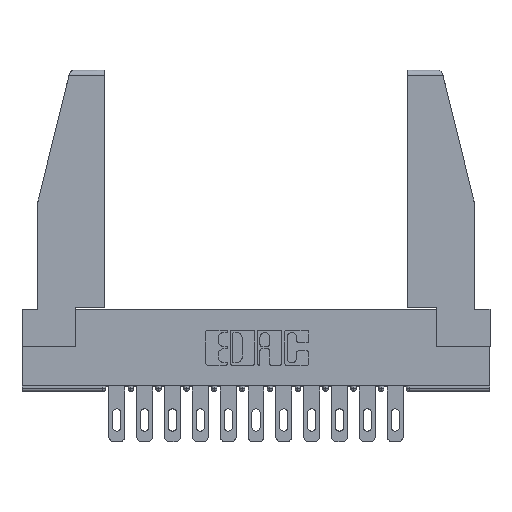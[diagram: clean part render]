
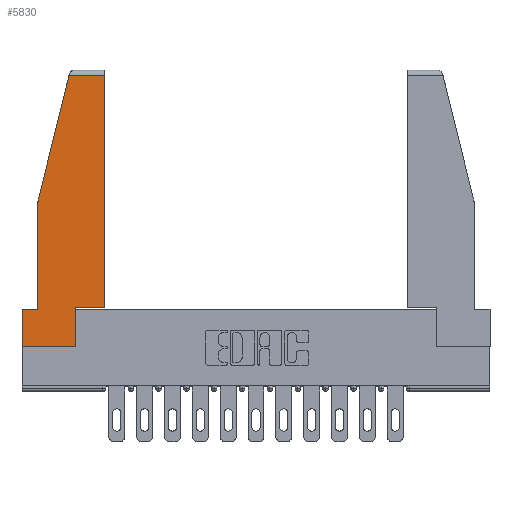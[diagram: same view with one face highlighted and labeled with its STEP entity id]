
A CAD part, top view. The second image highlights one B-rep face of the part: STEP entity #5830.
In plain terms, the highlighted planar face has unit normal (0, 0, 1).
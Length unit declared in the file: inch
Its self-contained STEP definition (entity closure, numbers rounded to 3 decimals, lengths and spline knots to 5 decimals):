
#15 = EDGE_CURVE ( 'NONE', #6433, #5348, #11458, .T. ) ;
#330 = DIRECTION ( 'NONE',  ( -1., 0., 0. ) ) ;
#631 = CARTESIAN_POINT ( 'NONE',  ( 0.297, 0., 0. ) ) ;
#1104 = DIRECTION ( 'NONE',  ( 1., 0., 0. ) ) ;
#1249 = ORIENTED_EDGE ( 'NONE', *, *, #12569, .T. ) ;
#1342 = CARTESIAN_POINT ( 'NONE',  ( 0., 0.21, 0. ) ) ;
#1896 = ORIENTED_EDGE ( 'NONE', *, *, #3203, .T. ) ;
#2034 = VECTOR ( 'NONE', #15187, 39.37008 ) ;
#2132 = VERTEX_POINT ( 'NONE', #4320 ) ;
#2552 = LINE ( 'NONE', #7394, #5013 ) ;
#2830 = VECTOR ( 'NONE', #11632, 39.37008 ) ;
#2908 = LINE ( 'NONE', #9413, #16476 ) ;
#3203 = EDGE_CURVE ( 'NONE', #11851, #7117, #3921, .T. ) ;
#3472 = VECTOR ( 'NONE', #7730, 39.37008 ) ;
#3849 = AXIS2_PLACEMENT_3D ( 'NONE', #8114, #9513, #1104 ) ;
#3921 = LINE ( 'NONE', #13723, #15728 ) ;
#4055 = EDGE_LOOP ( 'NONE', ( #10282, #1896, #13260, #15334, #10224, #13659, #14920, #1249, #7175 ) ) ;
#4320 = CARTESIAN_POINT ( 'NONE',  ( 0.297, 0., 0. ) ) ;
#4621 = VECTOR ( 'NONE', #14082, 39.37008 ) ;
#4877 = CARTESIAN_POINT ( 'NONE',  ( 0.461, 0.223, 0. ) ) ;
#5013 = VECTOR ( 'NONE', #330, 39.37008 ) ;
#5178 = CARTESIAN_POINT ( 'NONE',  ( 0.297, 0.223, 0. ) ) ;
#5245 = VERTEX_POINT ( 'NONE', #5178 ) ;
#5348 = VERTEX_POINT ( 'NONE', #12606 ) ;
#5524 = VECTOR ( 'NONE', #9646, 39.37008 ) ;
#5820 = CARTESIAN_POINT ( 'NONE',  ( 0.2636, 1.52, 0. ) ) ;
#5830 = ADVANCED_FACE ( 'NONE', ( #17944 ), #6725, .T. ) ;
#6433 = VERTEX_POINT ( 'NONE', #1342 ) ;
#6725 = PLANE ( 'NONE',  #3849 ) ;
#7117 = VERTEX_POINT ( 'NONE', #5820 ) ;
#7175 = ORIENTED_EDGE ( 'NONE', *, *, #15026, .T. ) ;
#7382 = CARTESIAN_POINT ( 'NONE',  ( 0.086, 0.8, 0. ) ) ;
#7394 = CARTESIAN_POINT ( 'NONE',  ( 0., 0.21, 0. ) ) ;
#7730 = DIRECTION ( 'NONE',  ( 0., -1., 0. ) ) ;
#8114 = CARTESIAN_POINT ( 'NONE',  ( 0., 0., 0. ) ) ;
#8249 = CARTESIAN_POINT ( 'NONE',  ( 0.297, 0.223, 0. ) ) ;
#8479 = EDGE_CURVE ( 'NONE', #7117, #10100, #2908, .T. ) ;
#8643 = VERTEX_POINT ( 'NONE', #9326 ) ;
#8775 = CARTESIAN_POINT ( 'NONE',  ( 0.461, 0.223, 0. ) ) ;
#9326 = CARTESIAN_POINT ( 'NONE',  ( 0.086, 0.21, 0. ) ) ;
#9413 = CARTESIAN_POINT ( 'NONE',  ( 0.271, 1.55, 0. ) ) ;
#9513 = DIRECTION ( 'NONE',  ( 0., 0., 1. ) ) ;
#9646 = DIRECTION ( 'NONE',  ( 1., 0., 0. ) ) ;
#10100 = VERTEX_POINT ( 'NONE', #7382 ) ;
#10139 = EDGE_CURVE ( 'NONE', #17479, #11851, #10907, .T. ) ;
#10224 = ORIENTED_EDGE ( 'NONE', *, *, #11218, .T. ) ;
#10282 = ORIENTED_EDGE ( 'NONE', *, *, #10139, .T. ) ;
#10804 = LINE ( 'NONE', #631, #12809 ) ;
#10900 = EDGE_CURVE ( 'NONE', #10100, #8643, #13528, .T. ) ;
#10907 = LINE ( 'NONE', #8775, #2830 ) ;
#11218 = EDGE_CURVE ( 'NONE', #8643, #6433, #2552, .T. ) ;
#11458 = LINE ( 'NONE', #13712, #2034 ) ;
#11632 = DIRECTION ( 'NONE',  ( 0., 1., 0. ) ) ;
#11851 = VERTEX_POINT ( 'NONE', #15563 ) ;
#12170 = DIRECTION ( 'NONE',  ( -0.239, -0.971, 0. ) ) ;
#12569 = EDGE_CURVE ( 'NONE', #2132, #5245, #10804, .T. ) ;
#12606 = CARTESIAN_POINT ( 'NONE',  ( 0., 0., 0. ) ) ;
#12809 = VECTOR ( 'NONE', #17321, 39.37008 ) ;
#13260 = ORIENTED_EDGE ( 'NONE', *, *, #8479, .T. ) ;
#13528 = LINE ( 'NONE', #17694, #3472 ) ;
#13591 = LINE ( 'NONE', #8249, #5524 ) ;
#13659 = ORIENTED_EDGE ( 'NONE', *, *, #15, .T. ) ;
#13712 = CARTESIAN_POINT ( 'NONE',  ( 0., 0.21, 0. ) ) ;
#13723 = CARTESIAN_POINT ( 'NONE',  ( 0., 1.52, 0. ) ) ;
#14082 = DIRECTION ( 'NONE',  ( 1., 0., 0. ) ) ;
#14670 = LINE ( 'NONE', #18079, #4621 ) ;
#14920 = ORIENTED_EDGE ( 'NONE', *, *, #15820, .T. ) ;
#15026 = EDGE_CURVE ( 'NONE', #5245, #17479, #13591, .T. ) ;
#15081 = DIRECTION ( 'NONE',  ( -1., 0., 0. ) ) ;
#15187 = DIRECTION ( 'NONE',  ( 0., -1., 0. ) ) ;
#15334 = ORIENTED_EDGE ( 'NONE', *, *, #10900, .T. ) ;
#15563 = CARTESIAN_POINT ( 'NONE',  ( 0.461, 1.52, 0. ) ) ;
#15728 = VECTOR ( 'NONE', #15081, 39.37008 ) ;
#15820 = EDGE_CURVE ( 'NONE', #5348, #2132, #14670, .T. ) ;
#16476 = VECTOR ( 'NONE', #12170, 39.37008 ) ;
#17321 = DIRECTION ( 'NONE',  ( 0., 1., 0. ) ) ;
#17479 = VERTEX_POINT ( 'NONE', #4877 ) ;
#17694 = CARTESIAN_POINT ( 'NONE',  ( 0.086, 0.8, 0. ) ) ;
#17944 = FACE_OUTER_BOUND ( 'NONE', #4055, .T. ) ;
#18079 = CARTESIAN_POINT ( 'NONE',  ( 0., 0., 0. ) ) ;
